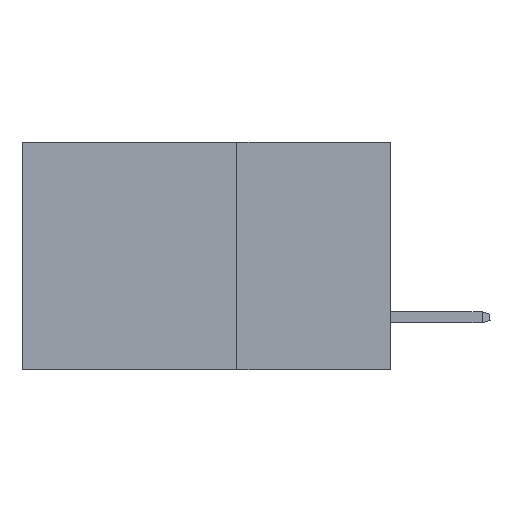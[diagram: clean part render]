
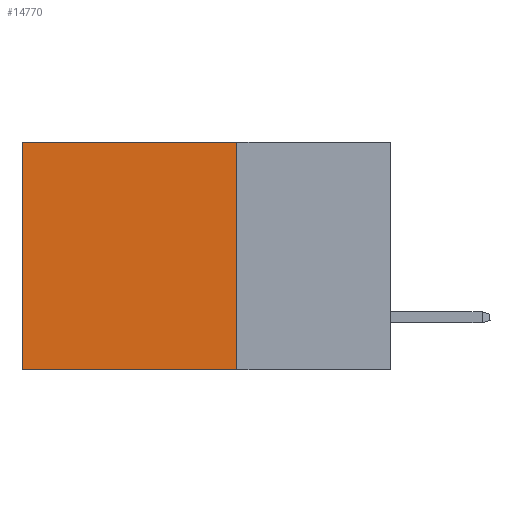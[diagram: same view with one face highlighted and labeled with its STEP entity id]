
A CAD part, left-side view. The second image highlights one B-rep face of the part: STEP entity #14770.
In plain terms, the highlighted planar face has unit normal (-1, 0, 0).
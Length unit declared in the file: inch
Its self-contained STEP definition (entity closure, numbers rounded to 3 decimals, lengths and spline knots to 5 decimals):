
#873 = DIRECTION ( 'NONE',  ( 1., 0., 0. ) ) ;
#2258 = EDGE_CURVE ( 'NONE', #14498, #21361, #17529, .T. ) ;
#2948 = EDGE_CURVE ( 'NONE', #16813, #21361, #22671, .T. ) ;
#3273 = VECTOR ( 'NONE', #17185, 39.37008 ) ;
#4656 = VECTOR ( 'NONE', #12169, 39.37008 ) ;
#8686 = EDGE_CURVE ( 'NONE', #17885, #16813, #16679, .T. ) ;
#9521 = VECTOR ( 'NONE', #10547, 39.37008 ) ;
#10277 = CARTESIAN_POINT ( 'NONE',  ( 0.2875, 0.6, 0. ) ) ;
#10547 = DIRECTION ( 'NONE',  ( 0., 1., 0. ) ) ;
#11119 = CARTESIAN_POINT ( 'NONE',  ( 0.2875, 0.6, -0.37 ) ) ;
#12057 = VECTOR ( 'NONE', #19162, 39.37008 ) ;
#12169 = DIRECTION ( 'NONE',  ( 0., 0., -1. ) ) ;
#12305 = CARTESIAN_POINT ( 'NONE',  ( 0.2875, 0.25, 0. ) ) ;
#12981 = LINE ( 'NONE', #21431, #9521 ) ;
#13260 = CARTESIAN_POINT ( 'NONE',  ( 0.2875, 0.25, 0. ) ) ;
#13583 = DIRECTION ( 'NONE',  ( 0., 0., -1. ) ) ;
#14498 = VERTEX_POINT ( 'NONE', #10277 ) ;
#14770 = ADVANCED_FACE ( 'NONE', ( #22480 ), #15378, .F. ) ;
#15347 = ORIENTED_EDGE ( 'NONE', *, *, #2258, .T. ) ;
#15353 = CARTESIAN_POINT ( 'NONE',  ( 0.2875, 0.25, -0.37 ) ) ;
#15378 = PLANE ( 'NONE',  #20761 ) ;
#15556 = ORIENTED_EDGE ( 'NONE', *, *, #23448, .T. ) ;
#15634 = CARTESIAN_POINT ( 'NONE',  ( 0.2875, 0.6, 0. ) ) ;
#15862 = ORIENTED_EDGE ( 'NONE', *, *, #2948, .F. ) ;
#16679 = LINE ( 'NONE', #21672, #4656 ) ;
#16813 = VERTEX_POINT ( 'NONE', #22877 ) ;
#17185 = DIRECTION ( 'NONE',  ( 0., 1., 0. ) ) ;
#17529 = LINE ( 'NONE', #15634, #12057 ) ;
#17885 = VERTEX_POINT ( 'NONE', #12305 ) ;
#19162 = DIRECTION ( 'NONE',  ( 0., 0., -1. ) ) ;
#20761 = AXIS2_PLACEMENT_3D ( 'NONE', #13260, #873, #13583 ) ;
#21361 = VERTEX_POINT ( 'NONE', #11119 ) ;
#21415 = ORIENTED_EDGE ( 'NONE', *, *, #8686, .F. ) ;
#21431 = CARTESIAN_POINT ( 'NONE',  ( 0.2875, 0.25, 0. ) ) ;
#21672 = CARTESIAN_POINT ( 'NONE',  ( 0.2875, 0.25, 0. ) ) ;
#22480 = FACE_OUTER_BOUND ( 'NONE', #23595, .T. ) ;
#22671 = LINE ( 'NONE', #15353, #3273 ) ;
#22877 = CARTESIAN_POINT ( 'NONE',  ( 0.2875, 0.25, -0.37 ) ) ;
#23448 = EDGE_CURVE ( 'NONE', #17885, #14498, #12981, .T. ) ;
#23595 = EDGE_LOOP ( 'NONE', ( #15347, #15862, #21415, #15556 ) ) ;
